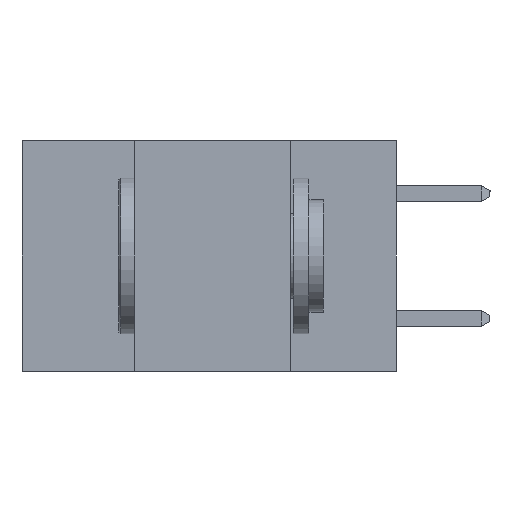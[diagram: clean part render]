
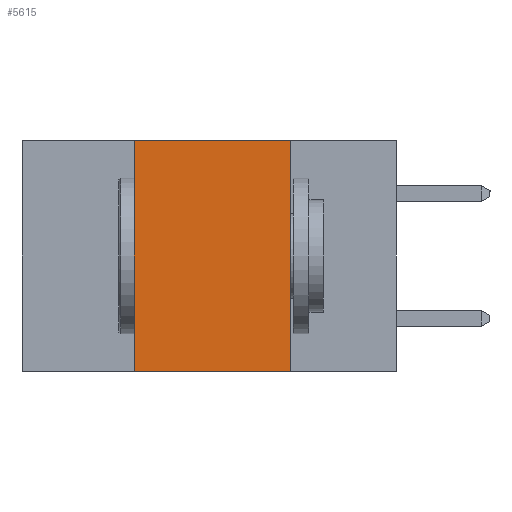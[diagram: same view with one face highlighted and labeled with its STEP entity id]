
A CAD part, left-side view. The second image highlights one B-rep face of the part: STEP entity #5615.
In plain terms, the highlighted planar face has unit normal (-1, 0, 0).
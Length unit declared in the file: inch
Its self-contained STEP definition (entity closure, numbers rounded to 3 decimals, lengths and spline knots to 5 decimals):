
#80 = CARTESIAN_POINT ( 'NONE',  ( 0., 0.17, -0.37 ) ) ;
#167 = VECTOR ( 'NONE', #2751, 39.37008 ) ;
#196 = EDGE_CURVE ( 'NONE', #3764, #9329, #1240, .T. ) ;
#213 = LINE ( 'NONE', #9016, #7042 ) ;
#609 = AXIS2_PLACEMENT_3D ( 'NONE', #2849, #2083, #7412 ) ;
#683 = DIRECTION ( 'NONE',  ( 0., -1., 0. ) ) ;
#736 = LINE ( 'NONE', #9078, #1943 ) ;
#1240 = LINE ( 'NONE', #9643, #167 ) ;
#1467 = EDGE_CURVE ( 'NONE', #3581, #7814, #6161, .T. ) ;
#1636 = CARTESIAN_POINT ( 'NONE',  ( 0., 0.42, 0. ) ) ;
#1676 = ORIENTED_EDGE ( 'NONE', *, *, #1467, .F. ) ;
#1943 = VECTOR ( 'NONE', #3813, 39.37008 ) ;
#2083 = DIRECTION ( 'NONE',  ( 1., 0., 0. ) ) ;
#2395 = DIRECTION ( 'NONE',  ( 0., 0., -1. ) ) ;
#2511 = CARTESIAN_POINT ( 'NONE',  ( 0., 0.17, 0. ) ) ;
#2688 = VECTOR ( 'NONE', #2395, 39.37008 ) ;
#2751 = DIRECTION ( 'NONE',  ( 0., 0., 1. ) ) ;
#2849 = CARTESIAN_POINT ( 'NONE',  ( 0., 0.6, 0. ) ) ;
#3159 = EDGE_LOOP ( 'NONE', ( #1676, #4173, #5770, #5567 ) ) ;
#3581 = VERTEX_POINT ( 'NONE', #2511 ) ;
#3764 = VERTEX_POINT ( 'NONE', #7664 ) ;
#3813 = DIRECTION ( 'NONE',  ( 0., -1., 0. ) ) ;
#4173 = ORIENTED_EDGE ( 'NONE', *, *, #9149, .F. ) ;
#5567 = ORIENTED_EDGE ( 'NONE', *, *, #7925, .T. ) ;
#5615 = ADVANCED_FACE ( 'NONE', ( #8114 ), #5918, .F. ) ;
#5770 = ORIENTED_EDGE ( 'NONE', *, *, #196, .F. ) ;
#5918 = PLANE ( 'NONE',  #609 ) ;
#6161 = LINE ( 'NONE', #80, #2688 ) ;
#6591 = CARTESIAN_POINT ( 'NONE',  ( 0., 0.17, -0.37 ) ) ;
#7042 = VECTOR ( 'NONE', #683, 39.37008 ) ;
#7412 = DIRECTION ( 'NONE',  ( 0., 0., -1. ) ) ;
#7664 = CARTESIAN_POINT ( 'NONE',  ( 0., 0.42, -0.37 ) ) ;
#7814 = VERTEX_POINT ( 'NONE', #6591 ) ;
#7925 = EDGE_CURVE ( 'NONE', #3764, #7814, #736, .T. ) ;
#8114 = FACE_OUTER_BOUND ( 'NONE', #3159, .T. ) ;
#9016 = CARTESIAN_POINT ( 'NONE',  ( 0., 0.6, 0. ) ) ;
#9078 = CARTESIAN_POINT ( 'NONE',  ( 0., 0.6, -0.37 ) ) ;
#9149 = EDGE_CURVE ( 'NONE', #9329, #3581, #213, .T. ) ;
#9329 = VERTEX_POINT ( 'NONE', #1636 ) ;
#9643 = CARTESIAN_POINT ( 'NONE',  ( 0., 0.42, -0.37 ) ) ;
